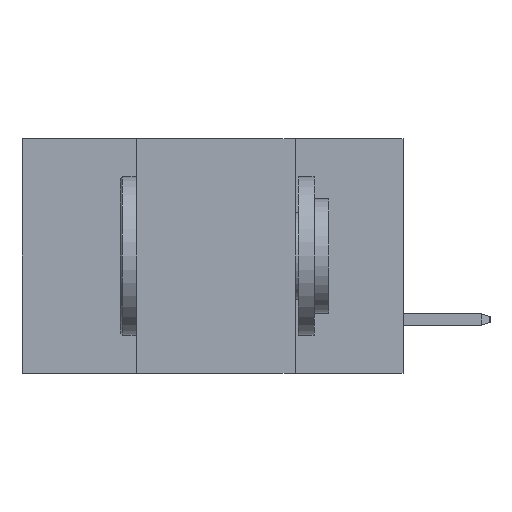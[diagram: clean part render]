
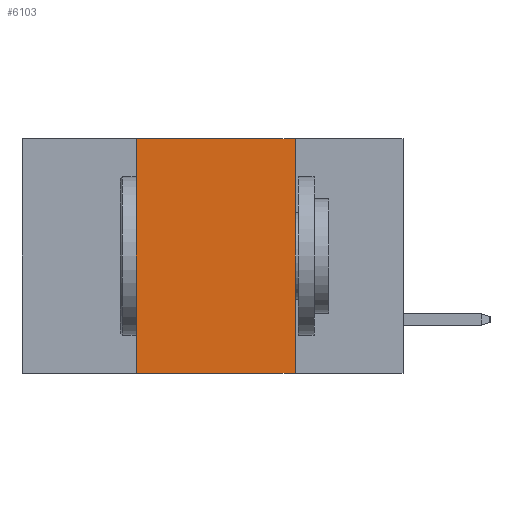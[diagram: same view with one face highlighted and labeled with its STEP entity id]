
A CAD part, left-side view. The second image highlights one B-rep face of the part: STEP entity #6103.
In plain terms, the highlighted planar face has unit normal (-1, 0, 0).
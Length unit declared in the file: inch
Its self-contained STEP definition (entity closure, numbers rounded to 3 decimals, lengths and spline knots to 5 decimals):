
#69 = VECTOR ( 'NONE', #3886, 39.37008 ) ;
#258 = LINE ( 'NONE', #5132, #4350 ) ;
#990 = DIRECTION ( 'NONE',  ( 0., 0., -1. ) ) ;
#1232 = FACE_OUTER_BOUND ( 'NONE', #12194, .T. ) ;
#1372 = CARTESIAN_POINT ( 'NONE',  ( 0., 0.17, -0.37 ) ) ;
#1616 = CARTESIAN_POINT ( 'NONE',  ( 0., 0.42, 0. ) ) ;
#2211 = VERTEX_POINT ( 'NONE', #1372 ) ;
#2440 = VERTEX_POINT ( 'NONE', #14531 ) ;
#2521 = LINE ( 'NONE', #5084, #69 ) ;
#2930 = LINE ( 'NONE', #13713, #3365 ) ;
#3365 = VECTOR ( 'NONE', #7664, 39.37008 ) ;
#3389 = PLANE ( 'NONE',  #3710 ) ;
#3710 = AXIS2_PLACEMENT_3D ( 'NONE', #9637, #8280, #990 ) ;
#3886 = DIRECTION ( 'NONE',  ( 0., -1., 0. ) ) ;
#4350 = VECTOR ( 'NONE', #6248, 39.37008 ) ;
#4741 = ORIENTED_EDGE ( 'NONE', *, *, #14416, .F. ) ;
#5084 = CARTESIAN_POINT ( 'NONE',  ( 0., 0.6, 0. ) ) ;
#5132 = CARTESIAN_POINT ( 'NONE',  ( 0., 0.6, -0.37 ) ) ;
#5557 = LINE ( 'NONE', #13942, #12970 ) ;
#6103 = ADVANCED_FACE ( 'NONE', ( #1232 ), #3389, .F. ) ;
#6248 = DIRECTION ( 'NONE',  ( 0., -1., 0. ) ) ;
#6648 = VERTEX_POINT ( 'NONE', #1616 ) ;
#6685 = DIRECTION ( 'NONE',  ( 0., 0., 1. ) ) ;
#7664 = DIRECTION ( 'NONE',  ( 0., 0., -1. ) ) ;
#8280 = DIRECTION ( 'NONE',  ( 1., 0., 0. ) ) ;
#8533 = EDGE_CURVE ( 'NONE', #2440, #6648, #5557, .T. ) ;
#8708 = ORIENTED_EDGE ( 'NONE', *, *, #14941, .F. ) ;
#8848 = VERTEX_POINT ( 'NONE', #12494 ) ;
#9637 = CARTESIAN_POINT ( 'NONE',  ( 0., 0.6, 0. ) ) ;
#9668 = ORIENTED_EDGE ( 'NONE', *, *, #8533, .F. ) ;
#10516 = EDGE_CURVE ( 'NONE', #2440, #2211, #258, .T. ) ;
#11312 = ORIENTED_EDGE ( 'NONE', *, *, #10516, .T. ) ;
#12194 = EDGE_LOOP ( 'NONE', ( #4741, #8708, #9668, #11312 ) ) ;
#12494 = CARTESIAN_POINT ( 'NONE',  ( 0., 0.17, 0. ) ) ;
#12970 = VECTOR ( 'NONE', #6685, 39.37008 ) ;
#13713 = CARTESIAN_POINT ( 'NONE',  ( 0., 0.17, 0. ) ) ;
#13942 = CARTESIAN_POINT ( 'NONE',  ( 0., 0.42, 0. ) ) ;
#14416 = EDGE_CURVE ( 'NONE', #8848, #2211, #2930, .T. ) ;
#14531 = CARTESIAN_POINT ( 'NONE',  ( 0., 0.42, -0.37 ) ) ;
#14941 = EDGE_CURVE ( 'NONE', #6648, #8848, #2521, .T. ) ;
